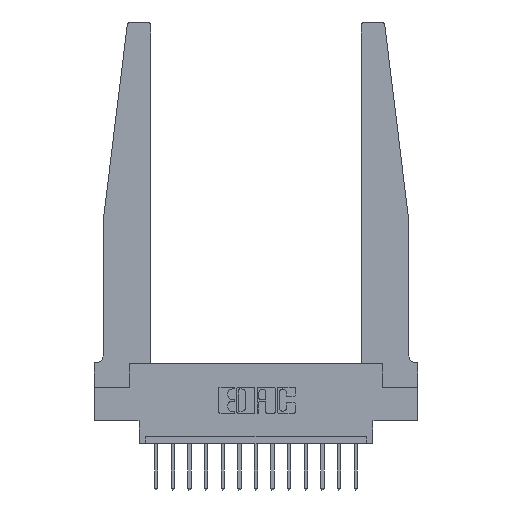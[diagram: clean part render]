
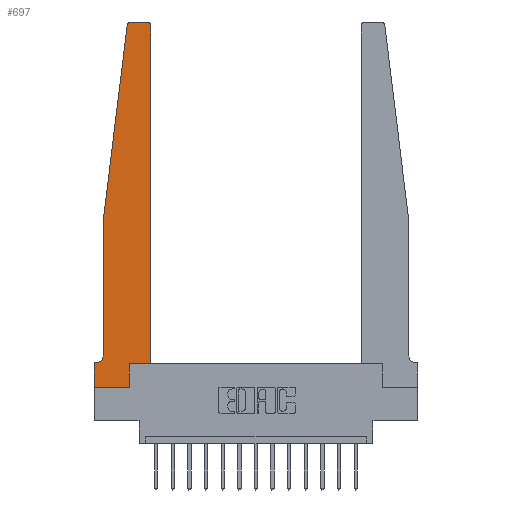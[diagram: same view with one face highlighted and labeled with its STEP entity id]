
A CAD part, top view. The second image highlights one B-rep face of the part: STEP entity #697.
In plain terms, the highlighted planar face has unit normal (0, 0, 1).
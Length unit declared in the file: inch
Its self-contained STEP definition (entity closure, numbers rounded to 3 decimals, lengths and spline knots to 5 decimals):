
#86 = VERTEX_POINT ( 'NONE', #15282 ) ;
#697 = ADVANCED_FACE ( 'NONE', ( #13232 ), #1215, .T. ) ;
#742 = VERTEX_POINT ( 'NONE', #10966 ) ;
#932 = VECTOR ( 'NONE', #15637, 39.37008 ) ;
#1040 = VECTOR ( 'NONE', #1557, 39.37008 ) ;
#1215 = PLANE ( 'NONE',  #4519 ) ;
#1305 = LINE ( 'NONE', #10877, #14327 ) ;
#1505 = ORIENTED_EDGE ( 'NONE', *, *, #8226, .T. ) ;
#1557 = DIRECTION ( 'NONE',  ( 0., 1., 0. ) ) ;
#1688 = CARTESIAN_POINT ( 'NONE',  ( 0.2605, 0.18, 0.37 ) ) ;
#2118 = AXIS2_PLACEMENT_3D ( 'NONE', #12209, #5424, #9384 ) ;
#2395 = CIRCLE ( 'NONE', #2118, 0.05 ) ;
#2436 = DIRECTION ( 'NONE',  ( 1., 0., 0. ) ) ;
#2528 = DIRECTION ( 'NONE',  ( 0., -1., 0. ) ) ;
#2864 = AXIS2_PLACEMENT_3D ( 'NONE', #6572, #9467, #11944 ) ;
#3600 = ORIENTED_EDGE ( 'NONE', *, *, #12833, .T. ) ;
#3710 = LINE ( 'NONE', #5192, #15278 ) ;
#4090 = LINE ( 'NONE', #13391, #16550 ) ;
#4354 = VECTOR ( 'NONE', #6553, 39.37008 ) ;
#4442 = VERTEX_POINT ( 'NONE', #12046 ) ;
#4506 = CARTESIAN_POINT ( 'NONE',  ( 0.27653, 2.75, 0.37 ) ) ;
#4519 = AXIS2_PLACEMENT_3D ( 'NONE', #13155, #6736, #2436 ) ;
#4530 = VERTEX_POINT ( 'NONE', #16475 ) ;
#4760 = CARTESIAN_POINT ( 'NONE',  ( 0.065, 1.25, 0.37 ) ) ;
#5192 = CARTESIAN_POINT ( 'NONE',  ( 0.065, 0.1875, 0.37 ) ) ;
#5226 = CARTESIAN_POINT ( 'NONE',  ( 0.2605, 0.18, 0.37 ) ) ;
#5355 = ORIENTED_EDGE ( 'NONE', *, *, #6634, .T. ) ;
#5424 = DIRECTION ( 'NONE',  ( 0., 0., -1. ) ) ;
#5715 = ORIENTED_EDGE ( 'NONE', *, *, #8950, .T. ) ;
#5850 = VECTOR ( 'NONE', #15914, 39.37008 ) ;
#5960 = CIRCLE ( 'NONE', #2864, 0.03 ) ;
#6211 = LINE ( 'NONE', #5226, #5850 ) ;
#6413 = ORIENTED_EDGE ( 'NONE', *, *, #8536, .T. ) ;
#6553 = DIRECTION ( 'NONE',  ( 1., 0., 0. ) ) ;
#6572 = CARTESIAN_POINT ( 'NONE',  ( 0.27653, 2.72, 0.37 ) ) ;
#6634 = EDGE_CURVE ( 'NONE', #86, #15810, #1305, .T. ) ;
#6736 = DIRECTION ( 'NONE',  ( 0., 0., 1. ) ) ;
#6747 = CARTESIAN_POINT ( 'NONE',  ( 0.065, 1.25, 0.37 ) ) ;
#7077 = VERTEX_POINT ( 'NONE', #1688 ) ;
#7235 = VERTEX_POINT ( 'NONE', #4506 ) ;
#7841 = EDGE_CURVE ( 'NONE', #7235, #8354, #5960, .T. ) ;
#8021 = AXIS2_PLACEMENT_3D ( 'NONE', #15682, #13067, #17158 ) ;
#8068 = LINE ( 'NONE', #14539, #4354 ) ;
#8185 = VECTOR ( 'NONE', #11909, 39.37008 ) ;
#8226 = EDGE_CURVE ( 'NONE', #4442, #7235, #4090, .T. ) ;
#8354 = VERTEX_POINT ( 'NONE', #14980 ) ;
#8536 = EDGE_CURVE ( 'NONE', #15810, #742, #13374, .T. ) ;
#8950 = EDGE_CURVE ( 'NONE', #9420, #10661, #13598, .T. ) ;
#9030 = ORIENTED_EDGE ( 'NONE', *, *, #16723, .T. ) ;
#9083 = DIRECTION ( 'NONE',  ( -1., 0., 0. ) ) ;
#9384 = DIRECTION ( 'NONE',  ( -1., 0., 0. ) ) ;
#9420 = VERTEX_POINT ( 'NONE', #11298 ) ;
#9426 = CARTESIAN_POINT ( 'NONE',  ( 0., 0., 0.37 ) ) ;
#9467 = DIRECTION ( 'NONE',  ( 0., 0., 1. ) ) ;
#9967 = CIRCLE ( 'NONE', #8021, 0.03 ) ;
#10243 = ORIENTED_EDGE ( 'NONE', *, *, #17071, .T. ) ;
#10292 = LINE ( 'NONE', #4760, #932 ) ;
#10389 = EDGE_CURVE ( 'NONE', #8354, #9420, #10292, .T. ) ;
#10661 = VERTEX_POINT ( 'NONE', #16474 ) ;
#10709 = VERTEX_POINT ( 'NONE', #13865 ) ;
#10877 = CARTESIAN_POINT ( 'NONE',  ( 0., 0., 0.37 ) ) ;
#10966 = CARTESIAN_POINT ( 'NONE',  ( 0.2605, 0., 0.37 ) ) ;
#11136 = VERTEX_POINT ( 'NONE', #11904 ) ;
#11298 = CARTESIAN_POINT ( 'NONE',  ( 0.065, 1.25, 0.37 ) ) ;
#11904 = CARTESIAN_POINT ( 'NONE',  ( 0.015, 0.1875, 0.37 ) ) ;
#11909 = DIRECTION ( 'NONE',  ( 1., 0., 0. ) ) ;
#11944 = DIRECTION ( 'NONE',  ( 1., 0., 0. ) ) ;
#12008 = DIRECTION ( 'NONE',  ( -1., 0., 0. ) ) ;
#12046 = CARTESIAN_POINT ( 'NONE',  ( 0.395, 2.75, 0.37 ) ) ;
#12111 = CARTESIAN_POINT ( 'NONE',  ( 0.425, 0.18, 0.37 ) ) ;
#12209 = CARTESIAN_POINT ( 'NONE',  ( 0.015, 0.2375, 0.37 ) ) ;
#12492 = CARTESIAN_POINT ( 'NONE',  ( 0., 0., 0.37 ) ) ;
#12604 = EDGE_CURVE ( 'NONE', #7077, #10709, #8068, .T. ) ;
#12833 = EDGE_CURVE ( 'NONE', #11136, #86, #3710, .T. ) ;
#12902 = EDGE_LOOP ( 'NONE', ( #1505, #16477, #13142, #5715, #14595, #3600, #5355, #6413, #10243, #16076, #9030, #14862 ) ) ;
#13067 = DIRECTION ( 'NONE',  ( 0., 0., 1. ) ) ;
#13142 = ORIENTED_EDGE ( 'NONE', *, *, #10389, .T. ) ;
#13155 = CARTESIAN_POINT ( 'NONE',  ( 0., 0.1875, 0.37 ) ) ;
#13232 = FACE_OUTER_BOUND ( 'NONE', #12902, .T. ) ;
#13306 = EDGE_CURVE ( 'NONE', #10661, #11136, #2395, .T. ) ;
#13329 = DIRECTION ( 'NONE',  ( 0., -1., 0. ) ) ;
#13374 = LINE ( 'NONE', #9426, #8185 ) ;
#13391 = CARTESIAN_POINT ( 'NONE',  ( 0.25, 2.75, 0.37 ) ) ;
#13547 = EDGE_CURVE ( 'NONE', #4530, #4442, #9967, .T. ) ;
#13583 = LINE ( 'NONE', #12111, #1040 ) ;
#13598 = LINE ( 'NONE', #6747, #15739 ) ;
#13865 = CARTESIAN_POINT ( 'NONE',  ( 0.425, 0.18, 0.37 ) ) ;
#14327 = VECTOR ( 'NONE', #2528, 39.37008 ) ;
#14539 = CARTESIAN_POINT ( 'NONE',  ( 0.425, 0.18, 0.37 ) ) ;
#14595 = ORIENTED_EDGE ( 'NONE', *, *, #13306, .T. ) ;
#14862 = ORIENTED_EDGE ( 'NONE', *, *, #13547, .T. ) ;
#14980 = CARTESIAN_POINT ( 'NONE',  ( 0.24675, 2.72367, 0.37 ) ) ;
#15278 = VECTOR ( 'NONE', #9083, 39.37008 ) ;
#15282 = CARTESIAN_POINT ( 'NONE',  ( 0., 0.1875, 0.37 ) ) ;
#15637 = DIRECTION ( 'NONE',  ( -0.122, -0.992, 0. ) ) ;
#15682 = CARTESIAN_POINT ( 'NONE',  ( 0.395, 2.72, 0.37 ) ) ;
#15739 = VECTOR ( 'NONE', #13329, 39.37008 ) ;
#15810 = VERTEX_POINT ( 'NONE', #12492 ) ;
#15914 = DIRECTION ( 'NONE',  ( 0., 1., 0. ) ) ;
#16076 = ORIENTED_EDGE ( 'NONE', *, *, #12604, .T. ) ;
#16474 = CARTESIAN_POINT ( 'NONE',  ( 0.065, 0.2375, 0.37 ) ) ;
#16475 = CARTESIAN_POINT ( 'NONE',  ( 0.425, 2.72, 0.37 ) ) ;
#16477 = ORIENTED_EDGE ( 'NONE', *, *, #7841, .T. ) ;
#16550 = VECTOR ( 'NONE', #12008, 39.37008 ) ;
#16723 = EDGE_CURVE ( 'NONE', #10709, #4530, #13583, .T. ) ;
#17071 = EDGE_CURVE ( 'NONE', #742, #7077, #6211, .T. ) ;
#17158 = DIRECTION ( 'NONE',  ( 1., 0., 0. ) ) ;
